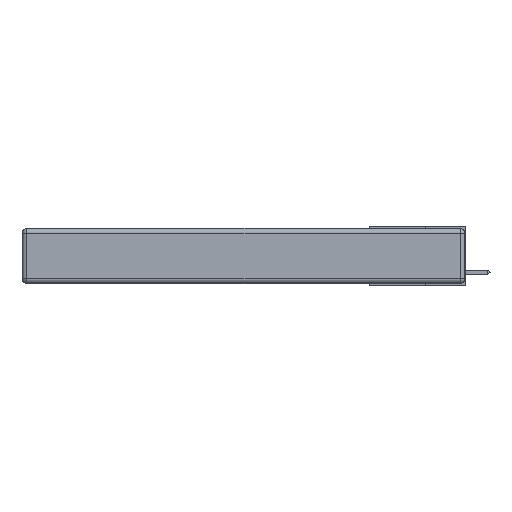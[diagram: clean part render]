
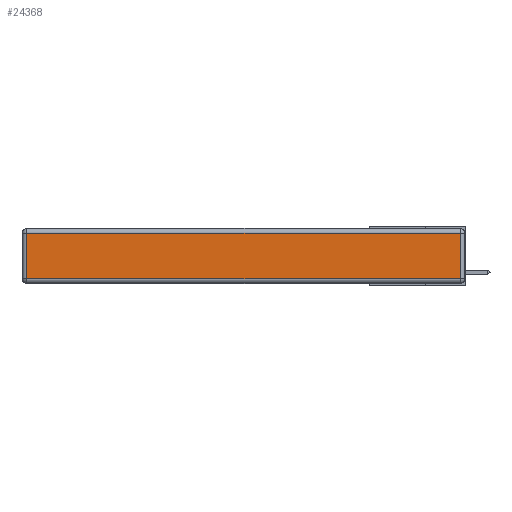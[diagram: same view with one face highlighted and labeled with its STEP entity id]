
A CAD part, left-side view. The second image highlights one B-rep face of the part: STEP entity #24368.
In plain terms, the highlighted planar face has unit normal (-1, 0, 0).
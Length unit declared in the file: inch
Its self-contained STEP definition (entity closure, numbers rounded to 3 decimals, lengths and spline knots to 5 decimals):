
#2492 = CARTESIAN_POINT ( 'NONE',  ( 0., 2.75, -0.03 ) ) ;
#3396 = PLANE ( 'NONE',  #30139 ) ;
#5275 = DIRECTION ( 'NONE',  ( 0., 0., -1. ) ) ;
#5741 = LINE ( 'NONE', #2492, #14345 ) ;
#9781 = EDGE_CURVE ( 'NONE', #16021, #10136, #5741, .T. ) ;
#10136 = VERTEX_POINT ( 'NONE', #30408 ) ;
#10244 = EDGE_CURVE ( 'NONE', #10136, #29515, #19126, .T. ) ;
#10880 = CARTESIAN_POINT ( 'NONE',  ( 0., 0., -0.343 ) ) ;
#10957 = LINE ( 'NONE', #30772, #12091 ) ;
#11311 = ORIENTED_EDGE ( 'NONE', *, *, #14693, .T. ) ;
#12091 = VECTOR ( 'NONE', #16486, 39.37008 ) ;
#12747 = CARTESIAN_POINT ( 'NONE',  ( 0., 0.03, -0.313 ) ) ;
#12948 = LINE ( 'NONE', #29606, #24877 ) ;
#13346 = ORIENTED_EDGE ( 'NONE', *, *, #16112, .T. ) ;
#14345 = VECTOR ( 'NONE', #19186, 39.37008 ) ;
#14693 = EDGE_CURVE ( 'NONE', #29515, #23724, #12948, .T. ) ;
#15292 = DIRECTION ( 'NONE',  ( -1., 0., 0. ) ) ;
#16021 = VERTEX_POINT ( 'NONE', #25519 ) ;
#16112 = EDGE_CURVE ( 'NONE', #23724, #16021, #10957, .T. ) ;
#16486 = DIRECTION ( 'NONE',  ( 0., 0., 1. ) ) ;
#16532 = VECTOR ( 'NONE', #5275, 39.37008 ) ;
#17671 = EDGE_LOOP ( 'NONE', ( #11311, #13346, #18515, #19332 ) ) ;
#18515 = ORIENTED_EDGE ( 'NONE', *, *, #9781, .T. ) ;
#19126 = LINE ( 'NONE', #19880, #16532 ) ;
#19186 = DIRECTION ( 'NONE',  ( 0., 1., 0. ) ) ;
#19332 = ORIENTED_EDGE ( 'NONE', *, *, #10244, .T. ) ;
#19880 = CARTESIAN_POINT ( 'NONE',  ( 0., 2.72, -0.343 ) ) ;
#20547 = FACE_OUTER_BOUND ( 'NONE', #17671, .T. ) ;
#23724 = VERTEX_POINT ( 'NONE', #12747 ) ;
#24368 = ADVANCED_FACE ( 'NONE', ( #20547 ), #3396, .T. ) ;
#24803 = DIRECTION ( 'NONE',  ( 0., -1., 0. ) ) ;
#24877 = VECTOR ( 'NONE', #24803, 39.37008 ) ;
#25519 = CARTESIAN_POINT ( 'NONE',  ( 0., 0.03, -0.03 ) ) ;
#25689 = DIRECTION ( 'NONE',  ( 0., 0., 1. ) ) ;
#29248 = CARTESIAN_POINT ( 'NONE',  ( 0., 2.72, -0.313 ) ) ;
#29515 = VERTEX_POINT ( 'NONE', #29248 ) ;
#29606 = CARTESIAN_POINT ( 'NONE',  ( 0., 0., -0.313 ) ) ;
#30139 = AXIS2_PLACEMENT_3D ( 'NONE', #10880, #15292, #25689 ) ;
#30408 = CARTESIAN_POINT ( 'NONE',  ( 0., 2.72, -0.03 ) ) ;
#30772 = CARTESIAN_POINT ( 'NONE',  ( 0., 0.03, -0.343 ) ) ;
